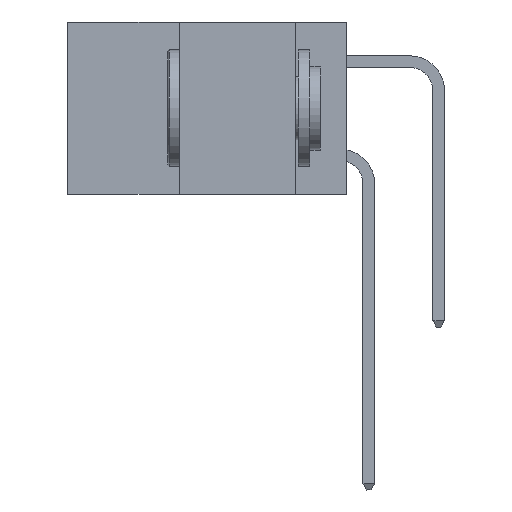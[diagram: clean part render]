
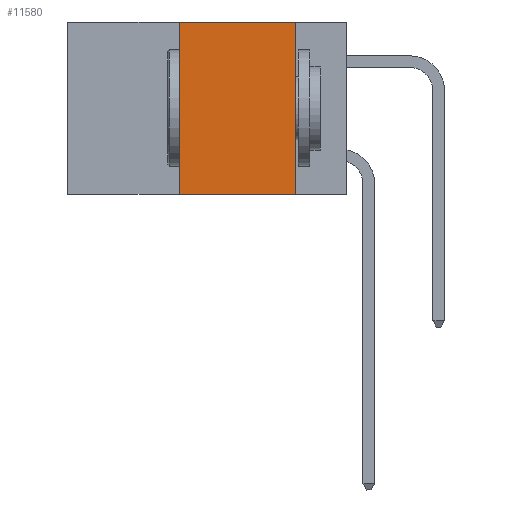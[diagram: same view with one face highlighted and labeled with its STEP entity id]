
A CAD part, left-side view. The second image highlights one B-rep face of the part: STEP entity #11580.
In plain terms, the highlighted planar face has unit normal (-1, 0, 0).
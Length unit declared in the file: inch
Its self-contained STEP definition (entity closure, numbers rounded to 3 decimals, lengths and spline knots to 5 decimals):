
#295 = VECTOR ( 'NONE', #4412, 39.37008 ) ;
#1274 = EDGE_CURVE ( 'NONE', #11829, #5423, #9337, .T. ) ;
#1286 = VECTOR ( 'NONE', #10723, 39.37008 ) ;
#1435 = VERTEX_POINT ( 'NONE', #9105 ) ;
#2475 = DIRECTION ( 'NONE',  ( 0., 0., 1. ) ) ;
#2493 = CARTESIAN_POINT ( 'NONE',  ( 0., 0.36, 0. ) ) ;
#2698 = CARTESIAN_POINT ( 'NONE',  ( 0., 0.6, 0. ) ) ;
#3489 = LINE ( 'NONE', #2493, #11648 ) ;
#4041 = EDGE_CURVE ( 'NONE', #11006, #11829, #3489, .T. ) ;
#4239 = LINE ( 'NONE', #9678, #1286 ) ;
#4412 = DIRECTION ( 'NONE',  ( 0., -1., 0. ) ) ;
#5027 = EDGE_LOOP ( 'NONE', ( #6460, #6761, #7155, #7846 ) ) ;
#5334 = CARTESIAN_POINT ( 'NONE',  ( 0., 0.6, -0.37 ) ) ;
#5423 = VERTEX_POINT ( 'NONE', #13118 ) ;
#5983 = PLANE ( 'NONE',  #6221 ) ;
#6076 = CARTESIAN_POINT ( 'NONE',  ( 0., 0.6, 0. ) ) ;
#6221 = AXIS2_PLACEMENT_3D ( 'NONE', #2698, #13367, #7090 ) ;
#6460 = ORIENTED_EDGE ( 'NONE', *, *, #7791, .F. ) ;
#6761 = ORIENTED_EDGE ( 'NONE', *, *, #1274, .F. ) ;
#7090 = DIRECTION ( 'NONE',  ( 0., 0., -1. ) ) ;
#7155 = ORIENTED_EDGE ( 'NONE', *, *, #4041, .F. ) ;
#7791 = EDGE_CURVE ( 'NONE', #5423, #1435, #4239, .T. ) ;
#7846 = ORIENTED_EDGE ( 'NONE', *, *, #8355, .T. ) ;
#8355 = EDGE_CURVE ( 'NONE', #11006, #1435, #10697, .T. ) ;
#9105 = CARTESIAN_POINT ( 'NONE',  ( 0., 0.11, -0.37 ) ) ;
#9337 = LINE ( 'NONE', #6076, #295 ) ;
#9678 = CARTESIAN_POINT ( 'NONE',  ( 0., 0.11, 0. ) ) ;
#10622 = DIRECTION ( 'NONE',  ( 0., -1., 0. ) ) ;
#10697 = LINE ( 'NONE', #5334, #13510 ) ;
#10723 = DIRECTION ( 'NONE',  ( 0., 0., -1. ) ) ;
#10775 = FACE_OUTER_BOUND ( 'NONE', #5027, .T. ) ;
#11006 = VERTEX_POINT ( 'NONE', #13431 ) ;
#11580 = ADVANCED_FACE ( 'NONE', ( #10775 ), #5983, .F. ) ;
#11648 = VECTOR ( 'NONE', #2475, 39.37008 ) ;
#11829 = VERTEX_POINT ( 'NONE', #13740 ) ;
#13118 = CARTESIAN_POINT ( 'NONE',  ( 0., 0.11, 0. ) ) ;
#13367 = DIRECTION ( 'NONE',  ( 1., 0., 0. ) ) ;
#13431 = CARTESIAN_POINT ( 'NONE',  ( 0., 0.36, -0.37 ) ) ;
#13510 = VECTOR ( 'NONE', #10622, 39.37008 ) ;
#13740 = CARTESIAN_POINT ( 'NONE',  ( 0., 0.36, 0. ) ) ;
